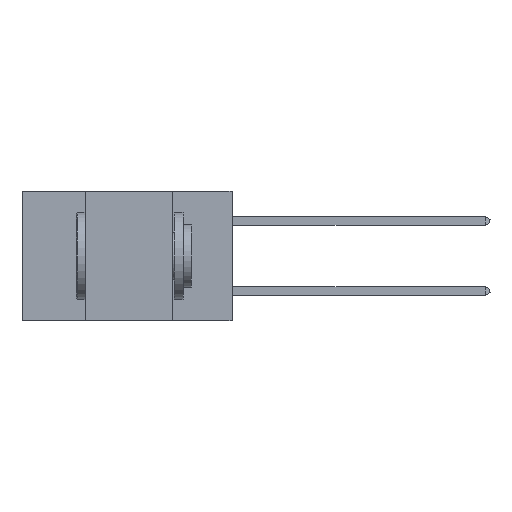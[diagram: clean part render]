
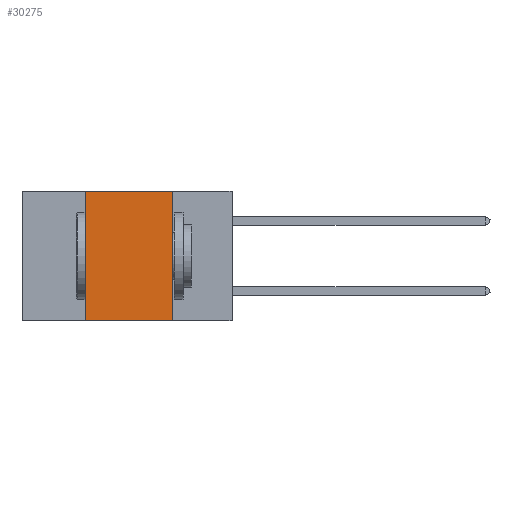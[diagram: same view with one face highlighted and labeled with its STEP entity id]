
A CAD part, left-side view. The second image highlights one B-rep face of the part: STEP entity #30275.
In plain terms, the highlighted planar face has unit normal (-1, 0, 0).
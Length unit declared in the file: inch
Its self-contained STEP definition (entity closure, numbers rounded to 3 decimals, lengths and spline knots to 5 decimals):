
#660 = CARTESIAN_POINT ( 'NONE',  ( 0., 0.42, -0.37 ) ) ;
#2825 = ORIENTED_EDGE ( 'NONE', *, *, #26803, .T. ) ;
#4612 = FACE_OUTER_BOUND ( 'NONE', #20642, .T. ) ;
#4659 = DIRECTION ( 'NONE',  ( 1., 0., 0. ) ) ;
#5385 = LINE ( 'NONE', #11861, #18912 ) ;
#6139 = AXIS2_PLACEMENT_3D ( 'NONE', #30199, #4659, #22614 ) ;
#6514 = CARTESIAN_POINT ( 'NONE',  ( 0., 0.42, 0. ) ) ;
#7030 = ORIENTED_EDGE ( 'NONE', *, *, #26538, .F. ) ;
#9707 = CARTESIAN_POINT ( 'NONE',  ( 0., 0.17, -0.37 ) ) ;
#9784 = VERTEX_POINT ( 'NONE', #6514 ) ;
#10829 = EDGE_CURVE ( 'NONE', #24850, #25607, #5385, .T. ) ;
#11585 = LINE ( 'NONE', #24494, #19963 ) ;
#11861 = CARTESIAN_POINT ( 'NONE',  ( 0., 0.17, 0. ) ) ;
#12354 = LINE ( 'NONE', #17834, #29859 ) ;
#12805 = DIRECTION ( 'NONE',  ( 0., -1., 0. ) ) ;
#13421 = EDGE_CURVE ( 'NONE', #19061, #9784, #21931, .T. ) ;
#14071 = ORIENTED_EDGE ( 'NONE', *, *, #10829, .F. ) ;
#14539 = DIRECTION ( 'NONE',  ( 0., 0., -1. ) ) ;
#15882 = DIRECTION ( 'NONE',  ( 0., 0., 1. ) ) ;
#16740 = DIRECTION ( 'NONE',  ( 0., -1., 0. ) ) ;
#17834 = CARTESIAN_POINT ( 'NONE',  ( 0., 0.6, -0.37 ) ) ;
#18912 = VECTOR ( 'NONE', #14539, 39.37008 ) ;
#19061 = VERTEX_POINT ( 'NONE', #660 ) ;
#19963 = VECTOR ( 'NONE', #16740, 39.37008 ) ;
#20642 = EDGE_LOOP ( 'NONE', ( #14071, #7030, #32269, #2825 ) ) ;
#21931 = LINE ( 'NONE', #31121, #22301 ) ;
#22301 = VECTOR ( 'NONE', #15882, 39.37008 ) ;
#22614 = DIRECTION ( 'NONE',  ( 0., 0., -1. ) ) ;
#24494 = CARTESIAN_POINT ( 'NONE',  ( 0., 0.6, 0. ) ) ;
#24850 = VERTEX_POINT ( 'NONE', #26302 ) ;
#25607 = VERTEX_POINT ( 'NONE', #9707 ) ;
#26302 = CARTESIAN_POINT ( 'NONE',  ( 0., 0.17, 0. ) ) ;
#26538 = EDGE_CURVE ( 'NONE', #9784, #24850, #11585, .T. ) ;
#26803 = EDGE_CURVE ( 'NONE', #19061, #25607, #12354, .T. ) ;
#29859 = VECTOR ( 'NONE', #12805, 39.37008 ) ;
#30199 = CARTESIAN_POINT ( 'NONE',  ( 0., 0.6, 0. ) ) ;
#30275 = ADVANCED_FACE ( 'NONE', ( #4612 ), #30531, .F. ) ;
#30531 = PLANE ( 'NONE',  #6139 ) ;
#31121 = CARTESIAN_POINT ( 'NONE',  ( 0., 0.42, 0. ) ) ;
#32269 = ORIENTED_EDGE ( 'NONE', *, *, #13421, .F. ) ;
